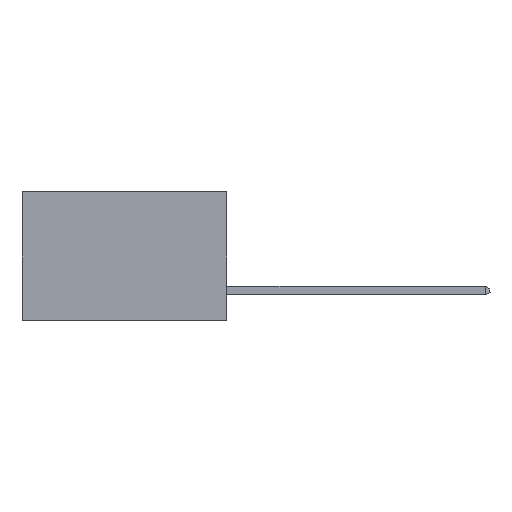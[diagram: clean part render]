
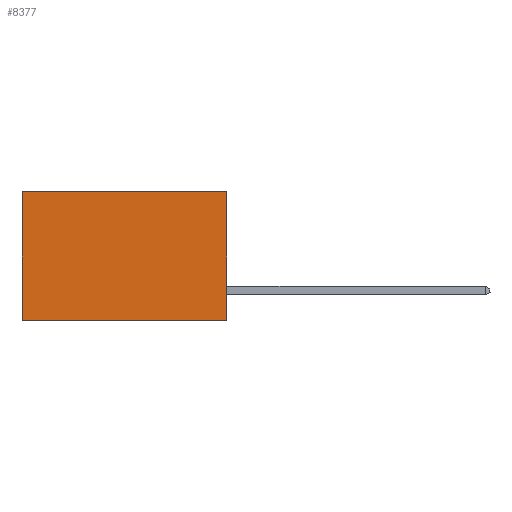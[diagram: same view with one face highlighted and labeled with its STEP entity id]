
A CAD part, left-side view. The second image highlights one B-rep face of the part: STEP entity #8377.
In plain terms, the highlighted planar face has unit normal (-1, 0, 0).
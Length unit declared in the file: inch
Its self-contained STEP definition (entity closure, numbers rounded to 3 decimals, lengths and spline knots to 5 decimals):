
#735 = VECTOR ( 'NONE', #1149, 39.37008 ) ;
#870 = DIRECTION ( 'NONE',  ( 0., 0., -1. ) ) ;
#1051 = PLANE ( 'NONE',  #12634 ) ;
#1149 = DIRECTION ( 'NONE',  ( 0., 0., -1. ) ) ;
#1157 = CARTESIAN_POINT ( 'NONE',  ( 0.277, 0., 0. ) ) ;
#2104 = VERTEX_POINT ( 'NONE', #3398 ) ;
#2126 = CARTESIAN_POINT ( 'NONE',  ( 0.277, 0.59, -0.37 ) ) ;
#2577 = LINE ( 'NONE', #1157, #15485 ) ;
#2754 = EDGE_CURVE ( 'NONE', #16101, #5666, #2577, .T. ) ;
#2916 = ORIENTED_EDGE ( 'NONE', *, *, #12878, .T. ) ;
#3398 = CARTESIAN_POINT ( 'NONE',  ( 0.277, 0., -0.37 ) ) ;
#3639 = EDGE_CURVE ( 'NONE', #2104, #12820, #9260, .T. ) ;
#4829 = LINE ( 'NONE', #16906, #11581 ) ;
#5038 = ORIENTED_EDGE ( 'NONE', *, *, #2754, .T. ) ;
#5666 = VERTEX_POINT ( 'NONE', #16969 ) ;
#5919 = DIRECTION ( 'NONE',  ( 0., 1., 0. ) ) ;
#7586 = LINE ( 'NONE', #7942, #735 ) ;
#7588 = ORIENTED_EDGE ( 'NONE', *, *, #15545, .F. ) ;
#7752 = DIRECTION ( 'NONE',  ( 0., 1., 0. ) ) ;
#7942 = CARTESIAN_POINT ( 'NONE',  ( 0.277, 0., -0.37 ) ) ;
#8307 = CARTESIAN_POINT ( 'NONE',  ( 0.277, 0., -0.37 ) ) ;
#8377 = ADVANCED_FACE ( 'NONE', ( #12925 ), #1051, .F. ) ;
#8833 = VECTOR ( 'NONE', #7752, 39.37008 ) ;
#9158 = EDGE_LOOP ( 'NONE', ( #2916, #14445, #7588, #5038 ) ) ;
#9245 = DIRECTION ( 'NONE',  ( 0., 0., -1. ) ) ;
#9260 = LINE ( 'NONE', #8307, #8833 ) ;
#11581 = VECTOR ( 'NONE', #870, 39.37008 ) ;
#12634 = AXIS2_PLACEMENT_3D ( 'NONE', #13194, #17129, #9245 ) ;
#12820 = VERTEX_POINT ( 'NONE', #2126 ) ;
#12878 = EDGE_CURVE ( 'NONE', #5666, #12820, #4829, .T. ) ;
#12925 = FACE_OUTER_BOUND ( 'NONE', #9158, .T. ) ;
#13194 = CARTESIAN_POINT ( 'NONE',  ( 0.277, 0., -0.37 ) ) ;
#14445 = ORIENTED_EDGE ( 'NONE', *, *, #3639, .F. ) ;
#15485 = VECTOR ( 'NONE', #5919, 39.37008 ) ;
#15545 = EDGE_CURVE ( 'NONE', #16101, #2104, #7586, .T. ) ;
#16101 = VERTEX_POINT ( 'NONE', #16409 ) ;
#16409 = CARTESIAN_POINT ( 'NONE',  ( 0.277, 0., 0. ) ) ;
#16906 = CARTESIAN_POINT ( 'NONE',  ( 0.277, 0.59, -0.37 ) ) ;
#16969 = CARTESIAN_POINT ( 'NONE',  ( 0.277, 0.59, 0. ) ) ;
#17129 = DIRECTION ( 'NONE',  ( 1., 0., 0. ) ) ;
